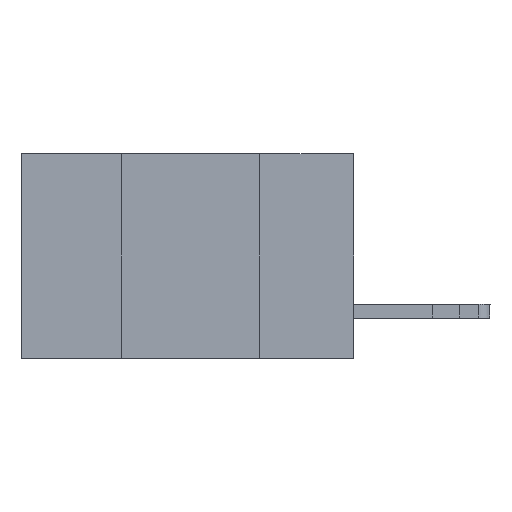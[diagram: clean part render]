
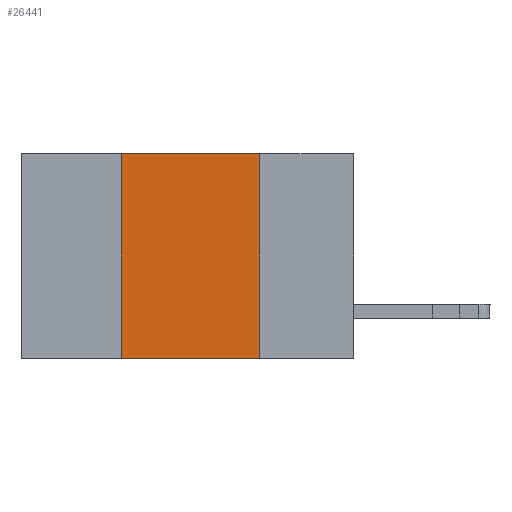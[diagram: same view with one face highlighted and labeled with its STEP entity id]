
A CAD part, left-side view. The second image highlights one B-rep face of the part: STEP entity #26441.
In plain terms, the highlighted planar face has unit normal (-1, 0, 0).
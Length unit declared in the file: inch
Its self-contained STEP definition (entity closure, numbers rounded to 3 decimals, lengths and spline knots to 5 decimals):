
#291 = EDGE_CURVE ( 'NONE', #17761, #26286, #17479, .T. ) ;
#783 = CARTESIAN_POINT ( 'NONE',  ( 0., 0.6, 0. ) ) ;
#1246 = VECTOR ( 'NONE', #28362, 39.37008 ) ;
#1880 = LINE ( 'NONE', #25620, #1246 ) ;
#1924 = CARTESIAN_POINT ( 'NONE',  ( 0., 0.17, -0.37 ) ) ;
#2547 = CARTESIAN_POINT ( 'NONE',  ( 0., 0.42, 0. ) ) ;
#4561 = PLANE ( 'NONE',  #13795 ) ;
#6367 = DIRECTION ( 'NONE',  ( 0., 0., 1. ) ) ;
#8905 = EDGE_CURVE ( 'NONE', #19534, #20741, #1880, .T. ) ;
#9314 = FACE_OUTER_BOUND ( 'NONE', #27449, .T. ) ;
#10418 = DIRECTION ( 'NONE',  ( 0., -1., 0. ) ) ;
#12256 = EDGE_CURVE ( 'NONE', #20741, #26286, #18320, .T. ) ;
#13009 = CARTESIAN_POINT ( 'NONE',  ( 0., 0.42, 0. ) ) ;
#13795 = AXIS2_PLACEMENT_3D ( 'NONE', #783, #13907, #26800 ) ;
#13813 = ORIENTED_EDGE ( 'NONE', *, *, #12256, .F. ) ;
#13907 = DIRECTION ( 'NONE',  ( 1., 0., 0. ) ) ;
#14515 = VECTOR ( 'NONE', #26607, 39.37008 ) ;
#14628 = ORIENTED_EDGE ( 'NONE', *, *, #28595, .F. ) ;
#14805 = ORIENTED_EDGE ( 'NONE', *, *, #291, .T. ) ;
#14878 = CARTESIAN_POINT ( 'NONE',  ( 0., 0.6, -0.37 ) ) ;
#17479 = LINE ( 'NONE', #14878, #22972 ) ;
#17761 = VERTEX_POINT ( 'NONE', #20263 ) ;
#18320 = LINE ( 'NONE', #20503, #14515 ) ;
#18512 = VECTOR ( 'NONE', #6367, 39.37008 ) ;
#19534 = VERTEX_POINT ( 'NONE', #2547 ) ;
#20263 = CARTESIAN_POINT ( 'NONE',  ( 0., 0.42, -0.37 ) ) ;
#20503 = CARTESIAN_POINT ( 'NONE',  ( 0., 0.17, 0. ) ) ;
#20741 = VERTEX_POINT ( 'NONE', #21912 ) ;
#21369 = LINE ( 'NONE', #13009, #18512 ) ;
#21912 = CARTESIAN_POINT ( 'NONE',  ( 0., 0.17, 0. ) ) ;
#22972 = VECTOR ( 'NONE', #10418, 39.37008 ) ;
#25186 = ORIENTED_EDGE ( 'NONE', *, *, #8905, .F. ) ;
#25620 = CARTESIAN_POINT ( 'NONE',  ( 0., 0.6, 0. ) ) ;
#26286 = VERTEX_POINT ( 'NONE', #1924 ) ;
#26441 = ADVANCED_FACE ( 'NONE', ( #9314 ), #4561, .F. ) ;
#26607 = DIRECTION ( 'NONE',  ( 0., 0., -1. ) ) ;
#26800 = DIRECTION ( 'NONE',  ( 0., 0., -1. ) ) ;
#27449 = EDGE_LOOP ( 'NONE', ( #13813, #25186, #14628, #14805 ) ) ;
#28362 = DIRECTION ( 'NONE',  ( 0., -1., 0. ) ) ;
#28595 = EDGE_CURVE ( 'NONE', #17761, #19534, #21369, .T. ) ;
